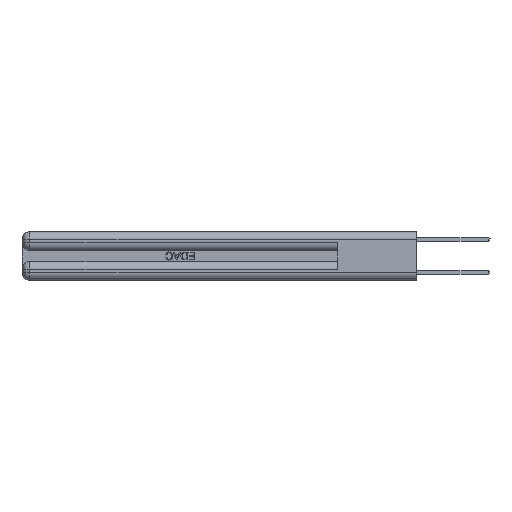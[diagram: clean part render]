
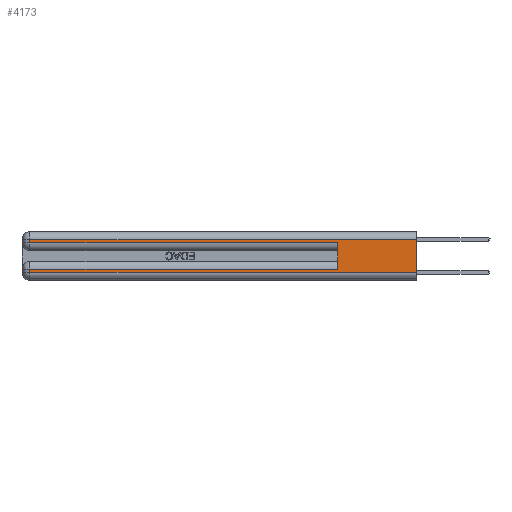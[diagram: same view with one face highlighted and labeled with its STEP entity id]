
A CAD part, left-side view. The second image highlights one B-rep face of the part: STEP entity #4173.
In plain terms, the highlighted planar face has unit normal (-1, 0, 0).
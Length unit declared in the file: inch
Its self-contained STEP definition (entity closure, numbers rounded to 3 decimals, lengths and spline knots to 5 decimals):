
#41 = CARTESIAN_POINT ( 'NONE',  ( 0., 0.6, 0.085 ) ) ;
#292 = VECTOR ( 'NONE', #21374, 39.37008 ) ;
#1174 = DIRECTION ( 'NONE',  ( 0., 0., -1. ) ) ;
#3058 = VERTEX_POINT ( 'NONE', #13273 ) ;
#3064 = CARTESIAN_POINT ( 'NONE',  ( 0., 0., 0.06 ) ) ;
#3442 = EDGE_CURVE ( 'NONE', #3058, #16307, #30039, .T. ) ;
#3685 = FACE_OUTER_BOUND ( 'NONE', #16608, .T. ) ;
#3848 = ORIENTED_EDGE ( 'NONE', *, *, #14782, .T. ) ;
#3991 = VERTEX_POINT ( 'NONE', #11950 ) ;
#4173 = ADVANCED_FACE ( 'NONE', ( #3685 ), #29003, .F. ) ;
#6171 = VECTOR ( 'NONE', #9082, 39.37008 ) ;
#6467 = EDGE_CURVE ( 'NONE', #28443, #28568, #23510, .T. ) ;
#7283 = VECTOR ( 'NONE', #23848, 39.37008 ) ;
#8385 = ORIENTED_EDGE ( 'NONE', *, *, #18615, .T. ) ;
#9020 = LINE ( 'NONE', #32771, #7283 ) ;
#9082 = DIRECTION ( 'NONE',  ( 0., 1., 0. ) ) ;
#9794 = DIRECTION ( 'NONE',  ( 0., -1., 0. ) ) ;
#10037 = VERTEX_POINT ( 'NONE', #19529 ) ;
#10354 = VECTOR ( 'NONE', #1174, 39.37008 ) ;
#10695 = VERTEX_POINT ( 'NONE', #41 ) ;
#11297 = DIRECTION ( 'NONE',  ( 0., -1., 0. ) ) ;
#11639 = CARTESIAN_POINT ( 'NONE',  ( 0., 0., 0.37 ) ) ;
#11950 = CARTESIAN_POINT ( 'NONE',  ( 0., 2.94, 0.085 ) ) ;
#12379 = DIRECTION ( 'NONE',  ( 0., 1., 0. ) ) ;
#13273 = CARTESIAN_POINT ( 'NONE',  ( 0., 2.94, 0.31 ) ) ;
#13682 = EDGE_CURVE ( 'NONE', #10695, #15873, #32290, .T. ) ;
#14440 = CARTESIAN_POINT ( 'NONE',  ( 0., 0., 0.06 ) ) ;
#14782 = EDGE_CURVE ( 'NONE', #16307, #15873, #35793, .T. ) ;
#14812 = CARTESIAN_POINT ( 'NONE',  ( 0., 0., 0.31 ) ) ;
#15873 = VERTEX_POINT ( 'NONE', #28816 ) ;
#16100 = VECTOR ( 'NONE', #22500, 39.37008 ) ;
#16222 = LINE ( 'NONE', #3064, #34616 ) ;
#16307 = VERTEX_POINT ( 'NONE', #33400 ) ;
#16608 = EDGE_LOOP ( 'NONE', ( #31070, #30829, #23312, #3848, #25767, #35126, #25658, #8385 ) ) ;
#17710 = CARTESIAN_POINT ( 'NONE',  ( 0., 0., 0.085 ) ) ;
#18615 = EDGE_CURVE ( 'NONE', #10037, #28568, #16222, .T. ) ;
#19529 = CARTESIAN_POINT ( 'NONE',  ( 0., 2.94, 0.06 ) ) ;
#20468 = VECTOR ( 'NONE', #12379, 39.37008 ) ;
#20865 = CARTESIAN_POINT ( 'NONE',  ( 0., 0., 0.285 ) ) ;
#21374 = DIRECTION ( 'NONE',  ( 0., 0., 1. ) ) ;
#22113 = EDGE_CURVE ( 'NONE', #28443, #3058, #26167, .T. ) ;
#22500 = DIRECTION ( 'NONE',  ( 0., 0., -1. ) ) ;
#23312 = ORIENTED_EDGE ( 'NONE', *, *, #3442, .T. ) ;
#23510 = LINE ( 'NONE', #11639, #16100 ) ;
#23784 = CARTESIAN_POINT ( 'NONE',  ( 0., 0., 0.37 ) ) ;
#23848 = DIRECTION ( 'NONE',  ( 0., 0., -1. ) ) ;
#25658 = ORIENTED_EDGE ( 'NONE', *, *, #26312, .T. ) ;
#25767 = ORIENTED_EDGE ( 'NONE', *, *, #13682, .F. ) ;
#25849 = LINE ( 'NONE', #17710, #6171 ) ;
#26167 = LINE ( 'NONE', #14812, #20468 ) ;
#26252 = CARTESIAN_POINT ( 'NONE',  ( 0., 0.6, 0.145 ) ) ;
#26312 = EDGE_CURVE ( 'NONE', #3991, #10037, #9020, .T. ) ;
#26369 = CARTESIAN_POINT ( 'NONE',  ( 0., 2.94, 0.37 ) ) ;
#27060 = AXIS2_PLACEMENT_3D ( 'NONE', #23784, #29131, #34557 ) ;
#28443 = VERTEX_POINT ( 'NONE', #29952 ) ;
#28568 = VERTEX_POINT ( 'NONE', #14440 ) ;
#28816 = CARTESIAN_POINT ( 'NONE',  ( 0., 0.6, 0.285 ) ) ;
#29003 = PLANE ( 'NONE',  #27060 ) ;
#29109 = VECTOR ( 'NONE', #9794, 39.37008 ) ;
#29131 = DIRECTION ( 'NONE',  ( 1., 0., 0. ) ) ;
#29952 = CARTESIAN_POINT ( 'NONE',  ( 0., 0., 0.31 ) ) ;
#30039 = LINE ( 'NONE', #26369, #10354 ) ;
#30829 = ORIENTED_EDGE ( 'NONE', *, *, #22113, .T. ) ;
#31070 = ORIENTED_EDGE ( 'NONE', *, *, #6467, .F. ) ;
#32290 = LINE ( 'NONE', #26252, #292 ) ;
#32771 = CARTESIAN_POINT ( 'NONE',  ( 0., 2.94, 0.37 ) ) ;
#33400 = CARTESIAN_POINT ( 'NONE',  ( 0., 2.94, 0.285 ) ) ;
#34033 = EDGE_CURVE ( 'NONE', #10695, #3991, #25849, .T. ) ;
#34557 = DIRECTION ( 'NONE',  ( 0., 0., -1. ) ) ;
#34616 = VECTOR ( 'NONE', #11297, 39.37008 ) ;
#35126 = ORIENTED_EDGE ( 'NONE', *, *, #34033, .T. ) ;
#35793 = LINE ( 'NONE', #20865, #29109 ) ;
